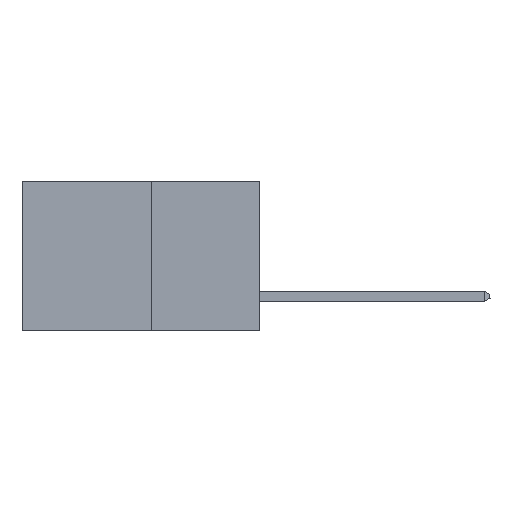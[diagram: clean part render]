
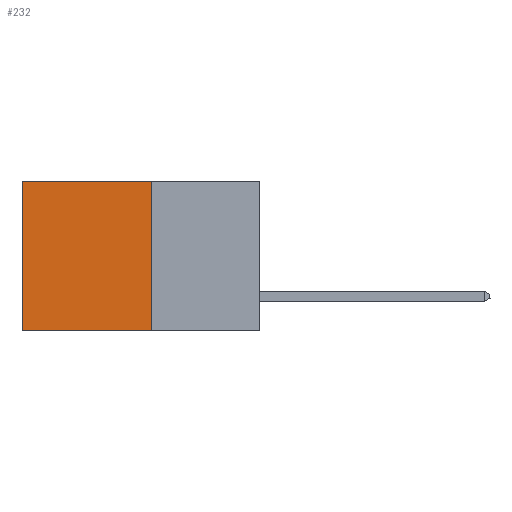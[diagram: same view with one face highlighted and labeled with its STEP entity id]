
A CAD part, left-side view. The second image highlights one B-rep face of the part: STEP entity #232.
In plain terms, the highlighted planar face has unit normal (-1, 0, 0).
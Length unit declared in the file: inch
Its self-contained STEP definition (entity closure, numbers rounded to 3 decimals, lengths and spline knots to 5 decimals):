
#232 = ADVANCED_FACE ( 'NONE', ( #5973 ), #10241, .F. ) ;
#266 = DIRECTION ( 'NONE',  ( 0., 1., 0. ) ) ;
#323 = ORIENTED_EDGE ( 'NONE', *, *, #13381, .F. ) ;
#2524 = CARTESIAN_POINT ( 'NONE',  ( 0.277, 0.27, -0.37 ) ) ;
#3451 = CARTESIAN_POINT ( 'NONE',  ( 0.277, 0.59, 0. ) ) ;
#3465 = CARTESIAN_POINT ( 'NONE',  ( 0.277, 0.27, -0.37 ) ) ;
#3543 = VECTOR ( 'NONE', #12601, 39.37008 ) ;
#4130 = CARTESIAN_POINT ( 'NONE',  ( 0.277, 0.27, -0.37 ) ) ;
#4729 = VECTOR ( 'NONE', #11156, 39.37008 ) ;
#5207 = ORIENTED_EDGE ( 'NONE', *, *, #8398, .T. ) ;
#5916 = VECTOR ( 'NONE', #17157, 39.37008 ) ;
#5973 = FACE_OUTER_BOUND ( 'NONE', #13353, .T. ) ;
#7188 = VECTOR ( 'NONE', #266, 39.37008 ) ;
#7496 = LINE ( 'NONE', #18243, #3543 ) ;
#8246 = ORIENTED_EDGE ( 'NONE', *, *, #8547, .F. ) ;
#8398 = EDGE_CURVE ( 'NONE', #15590, #11584, #8652, .T. ) ;
#8547 = EDGE_CURVE ( 'NONE', #15590, #14323, #10267, .T. ) ;
#8652 = LINE ( 'NONE', #18262, #4729 ) ;
#9008 = CARTESIAN_POINT ( 'NONE',  ( 0.277, 0.59, -0.37 ) ) ;
#9076 = CARTESIAN_POINT ( 'NONE',  ( 0.277, 0.27, -0.37 ) ) ;
#9084 = EDGE_CURVE ( 'NONE', #11584, #17097, #7496, .T. ) ;
#10241 = PLANE ( 'NONE',  #11086 ) ;
#10267 = LINE ( 'NONE', #2524, #5916 ) ;
#10285 = CARTESIAN_POINT ( 'NONE',  ( 0.277, 0.27, 0. ) ) ;
#10345 = DIRECTION ( 'NONE',  ( 0., 0., -1. ) ) ;
#10439 = DIRECTION ( 'NONE',  ( 1., 0., 0. ) ) ;
#10637 = LINE ( 'NONE', #9076, #7188 ) ;
#11086 = AXIS2_PLACEMENT_3D ( 'NONE', #3465, #10439, #10345 ) ;
#11156 = DIRECTION ( 'NONE',  ( 0., 1., 0. ) ) ;
#11584 = VERTEX_POINT ( 'NONE', #3451 ) ;
#12601 = DIRECTION ( 'NONE',  ( 0., 0., -1. ) ) ;
#13353 = EDGE_LOOP ( 'NONE', ( #13912, #323, #8246, #5207 ) ) ;
#13381 = EDGE_CURVE ( 'NONE', #14323, #17097, #10637, .T. ) ;
#13912 = ORIENTED_EDGE ( 'NONE', *, *, #9084, .T. ) ;
#14323 = VERTEX_POINT ( 'NONE', #4130 ) ;
#15590 = VERTEX_POINT ( 'NONE', #10285 ) ;
#17097 = VERTEX_POINT ( 'NONE', #9008 ) ;
#17157 = DIRECTION ( 'NONE',  ( 0., 0., -1. ) ) ;
#18243 = CARTESIAN_POINT ( 'NONE',  ( 0.277, 0.59, -0.37 ) ) ;
#18262 = CARTESIAN_POINT ( 'NONE',  ( 0.277, 0.27, 0. ) ) ;
